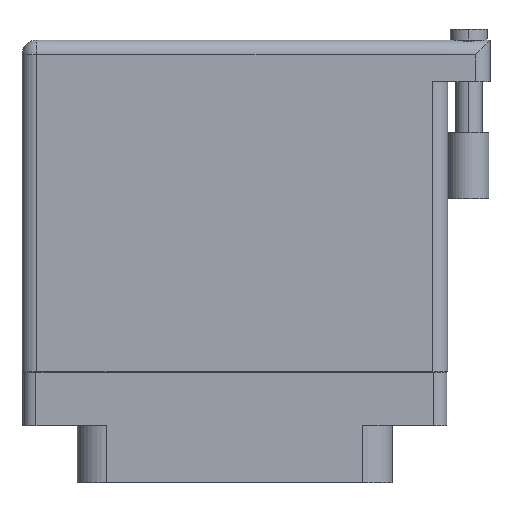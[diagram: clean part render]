
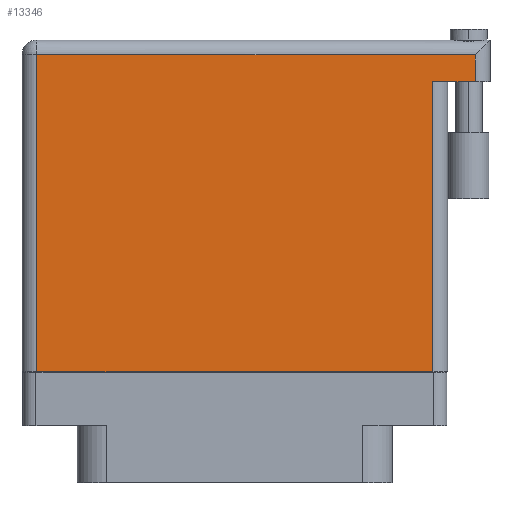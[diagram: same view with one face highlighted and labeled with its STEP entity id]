
A CAD part, front view. The second image highlights one B-rep face of the part: STEP entity #13346.
In plain terms, the highlighted face is planar.
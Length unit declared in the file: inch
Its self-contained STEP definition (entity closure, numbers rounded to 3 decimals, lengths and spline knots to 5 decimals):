
#105 = CARTESIAN_POINT ( 'NONE',  ( -0.934, -0.1, 0.4495 ) ) ;
#153 = EDGE_CURVE ( 'NONE', #28675, #28736, #21913, .T. ) ;
#343 = CARTESIAN_POINT ( 'NONE',  ( 0.934, 1.269, 0.4495 ) ) ;
#1167 = VECTOR ( 'NONE', #11556, 39.37008 ) ;
#1249 = ORIENTED_EDGE ( 'NONE', *, *, #25317, .T. ) ;
#1497 = CARTESIAN_POINT ( 'NONE',  ( 1.134, 1.269, 0.4495 ) ) ;
#2218 = CARTESIAN_POINT ( 'NONE',  ( -1.004, -0.1, 0.4495 ) ) ;
#3231 = EDGE_CURVE ( 'NONE', #16593, #8298, #34056, .T. ) ;
#4504 = CARTESIAN_POINT ( 'NONE',  ( 1.134, 1.396, 0.4495 ) ) ;
#5188 = DIRECTION ( 'NONE',  ( 0., 1., 0. ) ) ;
#5699 = EDGE_LOOP ( 'NONE', ( #14002, #1249, #15688, #16360, #14138, #31671 ) ) ;
#6320 = VECTOR ( 'NONE', #19641, 39.37008 ) ;
#7743 = VECTOR ( 'NONE', #27320, 39.37008 ) ;
#8182 = CARTESIAN_POINT ( 'NONE',  ( -0.934, -0.1, 0.4495 ) ) ;
#8298 = VERTEX_POINT ( 'NONE', #105 ) ;
#9071 = CARTESIAN_POINT ( 'NONE',  ( 0.934, -0.1, 0.4495 ) ) ;
#9272 = LINE ( 'NONE', #343, #6320 ) ;
#10077 = LINE ( 'NONE', #2218, #25648 ) ;
#10776 = EDGE_CURVE ( 'NONE', #28675, #21799, #30465, .T. ) ;
#11556 = DIRECTION ( 'NONE',  ( -1., 0., 0. ) ) ;
#13346 = ADVANCED_FACE ( 'NONE', ( #32045 ), #35128, .F. ) ;
#14002 = ORIENTED_EDGE ( 'NONE', *, *, #18525, .T. ) ;
#14138 = ORIENTED_EDGE ( 'NONE', *, *, #29646, .T. ) ;
#15231 = LINE ( 'NONE', #32971, #34226 ) ;
#15688 = ORIENTED_EDGE ( 'NONE', *, *, #10776, .F. ) ;
#16296 = DIRECTION ( 'NONE',  ( 1., 0., 0. ) ) ;
#16360 = ORIENTED_EDGE ( 'NONE', *, *, #153, .T. ) ;
#16593 = VERTEX_POINT ( 'NONE', #22888 ) ;
#18525 = EDGE_CURVE ( 'NONE', #8298, #29860, #10077, .T. ) ;
#19489 = DIRECTION ( 'NONE',  ( -1., 0., 0. ) ) ;
#19641 = DIRECTION ( 'NONE',  ( 0., 1., 0. ) ) ;
#21255 = DIRECTION ( 'NONE',  ( -1., 0., 0. ) ) ;
#21438 = VECTOR ( 'NONE', #5188, 39.37008 ) ;
#21799 = VERTEX_POINT ( 'NONE', #25524 ) ;
#21913 = LINE ( 'NONE', #33665, #21438 ) ;
#22888 = CARTESIAN_POINT ( 'NONE',  ( -0.934, 1.396, 0.4495 ) ) ;
#23926 = CARTESIAN_POINT ( 'NONE',  ( -1.004, 1.466, 0.4495 ) ) ;
#25317 = EDGE_CURVE ( 'NONE', #29860, #21799, #9272, .T. ) ;
#25524 = CARTESIAN_POINT ( 'NONE',  ( 0.934, 1.269, 0.4495 ) ) ;
#25541 = CARTESIAN_POINT ( 'NONE',  ( 1.204, 1.269, 0.4495 ) ) ;
#25648 = VECTOR ( 'NONE', #16296, 39.37008 ) ;
#26937 = DIRECTION ( 'NONE',  ( 0., 0., -1. ) ) ;
#27086 = AXIS2_PLACEMENT_3D ( 'NONE', #23926, #26937, #21255 ) ;
#27320 = DIRECTION ( 'NONE',  ( 0., -1., 0. ) ) ;
#28675 = VERTEX_POINT ( 'NONE', #1497 ) ;
#28736 = VERTEX_POINT ( 'NONE', #4504 ) ;
#29646 = EDGE_CURVE ( 'NONE', #28736, #16593, #15231, .T. ) ;
#29860 = VERTEX_POINT ( 'NONE', #9071 ) ;
#30465 = LINE ( 'NONE', #25541, #1167 ) ;
#31671 = ORIENTED_EDGE ( 'NONE', *, *, #3231, .T. ) ;
#32045 = FACE_OUTER_BOUND ( 'NONE', #5699, .T. ) ;
#32971 = CARTESIAN_POINT ( 'NONE',  ( -1.004, 1.396, 0.4495 ) ) ;
#33665 = CARTESIAN_POINT ( 'NONE',  ( 1.134, 1.466, 0.4495 ) ) ;
#34056 = LINE ( 'NONE', #8182, #7743 ) ;
#34226 = VECTOR ( 'NONE', #19489, 39.37008 ) ;
#35128 = PLANE ( 'NONE',  #27086 ) ;
